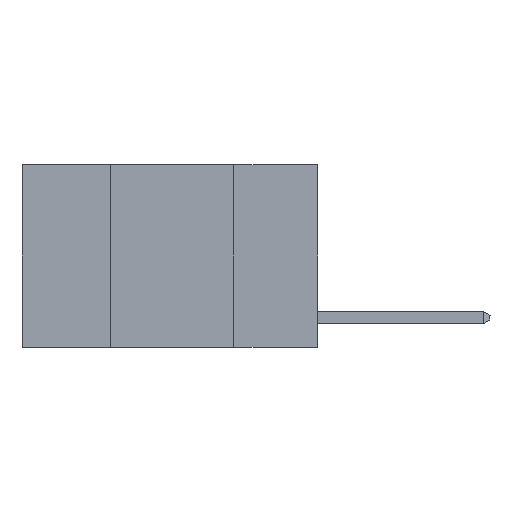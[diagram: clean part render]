
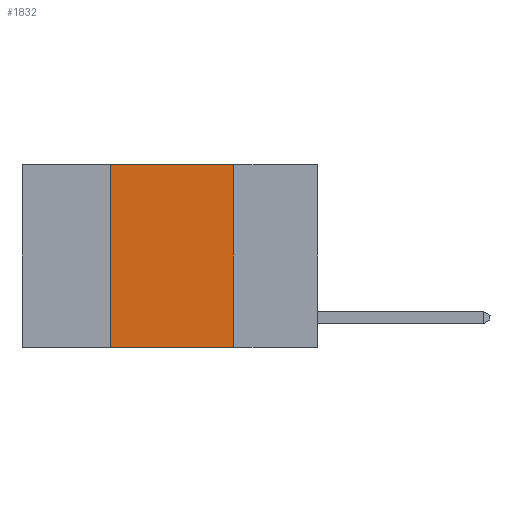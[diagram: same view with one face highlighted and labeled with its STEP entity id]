
A CAD part, left-side view. The second image highlights one B-rep face of the part: STEP entity #1832.
In plain terms, the highlighted planar face has unit normal (-1, 0, 0).
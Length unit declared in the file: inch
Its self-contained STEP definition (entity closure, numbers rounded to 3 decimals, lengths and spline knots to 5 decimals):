
#126 = CARTESIAN_POINT ( 'NONE',  ( 0., 0.17, 0. ) ) ;
#481 = DIRECTION ( 'NONE',  ( 0., 0., -1. ) ) ;
#486 = CARTESIAN_POINT ( 'NONE',  ( 0., 0.6, 0. ) ) ;
#537 = CARTESIAN_POINT ( 'NONE',  ( 0., 0.17, 0. ) ) ;
#588 = ORIENTED_EDGE ( 'NONE', *, *, #10598, .F. ) ;
#1228 = ORIENTED_EDGE ( 'NONE', *, *, #15941, .F. ) ;
#1556 = EDGE_CURVE ( 'NONE', #12301, #1857, #7420, .T. ) ;
#1832 = ADVANCED_FACE ( 'NONE', ( #8876 ), #1840, .F. ) ;
#1840 = PLANE ( 'NONE',  #8716 ) ;
#1857 = VERTEX_POINT ( 'NONE', #12382 ) ;
#2912 = CARTESIAN_POINT ( 'NONE',  ( 0., 0.42, 0. ) ) ;
#3014 = EDGE_LOOP ( 'NONE', ( #588, #15180, #1228, #13079 ) ) ;
#4107 = VECTOR ( 'NONE', #6257, 39.37008 ) ;
#5229 = LINE ( 'NONE', #10240, #9194 ) ;
#5318 = CARTESIAN_POINT ( 'NONE',  ( 0., 0.42, -0.37 ) ) ;
#5565 = LINE ( 'NONE', #537, #5961 ) ;
#5884 = DIRECTION ( 'NONE',  ( 0., 0., -1. ) ) ;
#5961 = VECTOR ( 'NONE', #481, 39.37008 ) ;
#6257 = DIRECTION ( 'NONE',  ( 0., -1., 0. ) ) ;
#6673 = LINE ( 'NONE', #486, #15702 ) ;
#7348 = VERTEX_POINT ( 'NONE', #2912 ) ;
#7420 = LINE ( 'NONE', #8995, #4107 ) ;
#7594 = DIRECTION ( 'NONE',  ( 0., 0., 1. ) ) ;
#8716 = AXIS2_PLACEMENT_3D ( 'NONE', #14886, #11056, #5884 ) ;
#8876 = FACE_OUTER_BOUND ( 'NONE', #3014, .T. ) ;
#8995 = CARTESIAN_POINT ( 'NONE',  ( 0., 0.6, -0.37 ) ) ;
#9194 = VECTOR ( 'NONE', #7594, 39.37008 ) ;
#10240 = CARTESIAN_POINT ( 'NONE',  ( 0., 0.42, 0. ) ) ;
#10598 = EDGE_CURVE ( 'NONE', #16512, #1857, #5565, .T. ) ;
#11056 = DIRECTION ( 'NONE',  ( 1., 0., 0. ) ) ;
#12301 = VERTEX_POINT ( 'NONE', #5318 ) ;
#12382 = CARTESIAN_POINT ( 'NONE',  ( 0., 0.17, -0.37 ) ) ;
#13079 = ORIENTED_EDGE ( 'NONE', *, *, #1556, .T. ) ;
#13380 = DIRECTION ( 'NONE',  ( 0., -1., 0. ) ) ;
#14886 = CARTESIAN_POINT ( 'NONE',  ( 0., 0.6, 0. ) ) ;
#15180 = ORIENTED_EDGE ( 'NONE', *, *, #15213, .F. ) ;
#15213 = EDGE_CURVE ( 'NONE', #7348, #16512, #6673, .T. ) ;
#15702 = VECTOR ( 'NONE', #13380, 39.37008 ) ;
#15941 = EDGE_CURVE ( 'NONE', #12301, #7348, #5229, .T. ) ;
#16512 = VERTEX_POINT ( 'NONE', #126 ) ;
